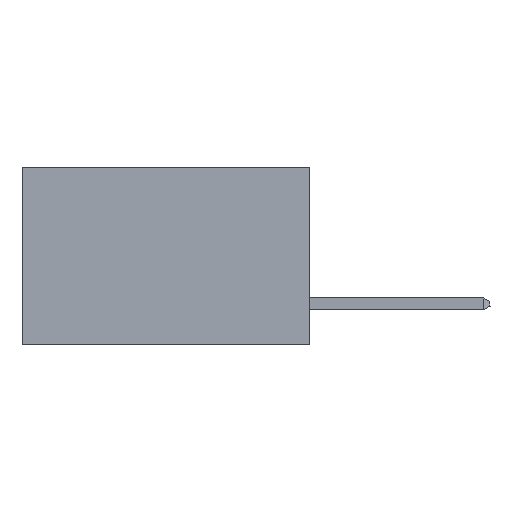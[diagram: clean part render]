
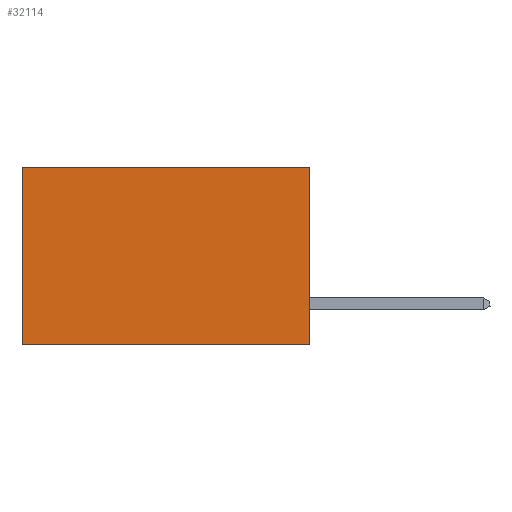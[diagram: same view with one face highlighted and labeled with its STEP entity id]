
A CAD part, left-side view. The second image highlights one B-rep face of the part: STEP entity #32114.
In plain terms, the highlighted planar face has unit normal (-1, 0, 0).
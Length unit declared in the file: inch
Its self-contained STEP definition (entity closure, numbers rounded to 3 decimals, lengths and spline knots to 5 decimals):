
#1913 = ORIENTED_EDGE ( 'NONE', *, *, #15670, .F. ) ;
#4829 = EDGE_LOOP ( 'NONE', ( #32367, #1913, #32532, #32403 ) ) ;
#6183 = EDGE_CURVE ( 'NONE', #17632, #46035, #34746, .T. ) ;
#6635 = VERTEX_POINT ( 'NONE', #23976 ) ;
#7686 = FACE_OUTER_BOUND ( 'NONE', #4829, .T. ) ;
#8333 = VECTOR ( 'NONE', #47058, 39.37008 ) ;
#9053 = DIRECTION ( 'NONE',  ( 0., 0., -1. ) ) ;
#11395 = LINE ( 'NONE', #26491, #45437 ) ;
#13234 = PLANE ( 'NONE',  #36577 ) ;
#13921 = EDGE_CURVE ( 'NONE', #17632, #6635, #11395, .T. ) ;
#15670 = EDGE_CURVE ( 'NONE', #6635, #26589, #42557, .T. ) ;
#16982 = DIRECTION ( 'NONE',  ( 0., 0., -1. ) ) ;
#17632 = VERTEX_POINT ( 'NONE', #28845 ) ;
#18795 = DIRECTION ( 'NONE',  ( 0., 1., 0. ) ) ;
#23466 = CARTESIAN_POINT ( 'NONE',  ( 0.2875, 0.6, -0.37 ) ) ;
#23789 = CARTESIAN_POINT ( 'NONE',  ( 0.2875, 0.6, 0. ) ) ;
#23976 = CARTESIAN_POINT ( 'NONE',  ( 0.2875, 0., -0.37 ) ) ;
#26491 = CARTESIAN_POINT ( 'NONE',  ( 0.2875, 0., 0. ) ) ;
#26589 = VERTEX_POINT ( 'NONE', #23466 ) ;
#28845 = CARTESIAN_POINT ( 'NONE',  ( 0.2875, 0., 0. ) ) ;
#32114 = ADVANCED_FACE ( 'NONE', ( #7686 ), #13234, .F. ) ;
#32367 = ORIENTED_EDGE ( 'NONE', *, *, #39878, .T. ) ;
#32403 = ORIENTED_EDGE ( 'NONE', *, *, #6183, .T. ) ;
#32532 = ORIENTED_EDGE ( 'NONE', *, *, #13921, .F. ) ;
#34078 = DIRECTION ( 'NONE',  ( 0., 0., -1. ) ) ;
#34746 = LINE ( 'NONE', #35560, #8333 ) ;
#35086 = DIRECTION ( 'NONE',  ( 1., 0., 0. ) ) ;
#35560 = CARTESIAN_POINT ( 'NONE',  ( 0.2875, 0., 0. ) ) ;
#36577 = AXIS2_PLACEMENT_3D ( 'NONE', #43122, #35086, #16982 ) ;
#37556 = CARTESIAN_POINT ( 'NONE',  ( 0.2875, 0., -0.37 ) ) ;
#38451 = VECTOR ( 'NONE', #18795, 39.37008 ) ;
#39878 = EDGE_CURVE ( 'NONE', #46035, #26589, #41542, .T. ) ;
#40543 = CARTESIAN_POINT ( 'NONE',  ( 0.2875, 0.6, 0. ) ) ;
#41542 = LINE ( 'NONE', #23789, #42717 ) ;
#42557 = LINE ( 'NONE', #37556, #38451 ) ;
#42717 = VECTOR ( 'NONE', #9053, 39.37008 ) ;
#43122 = CARTESIAN_POINT ( 'NONE',  ( 0.2875, 0., 0. ) ) ;
#45437 = VECTOR ( 'NONE', #34078, 39.37008 ) ;
#46035 = VERTEX_POINT ( 'NONE', #40543 ) ;
#47058 = DIRECTION ( 'NONE',  ( 0., 1., 0. ) ) ;
